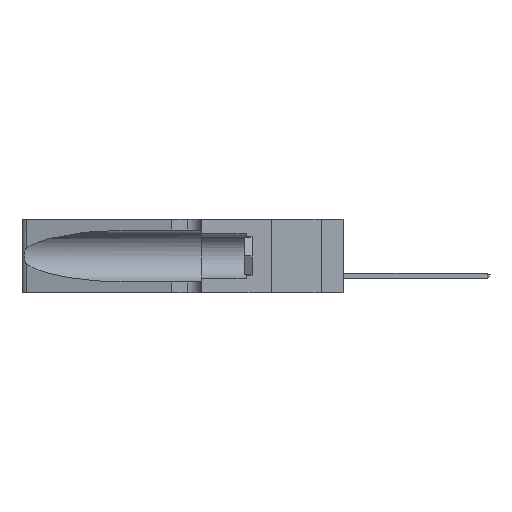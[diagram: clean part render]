
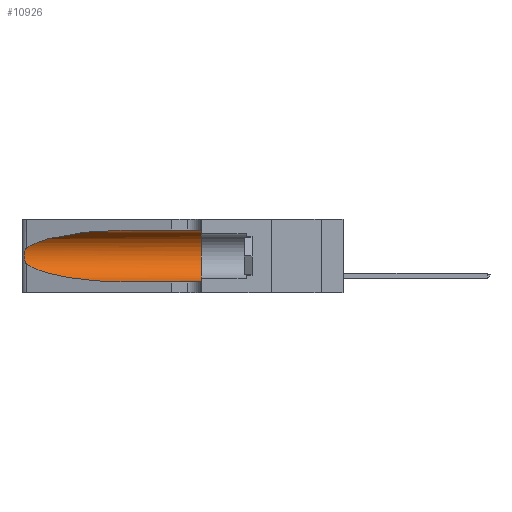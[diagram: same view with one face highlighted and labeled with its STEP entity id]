
A CAD part, left-side view. The second image highlights one B-rep face of the part: STEP entity #10926.
In plain terms, the highlighted cylindrical face has radius 3.308 mm (diameter 6.617 mm), a partial arc.
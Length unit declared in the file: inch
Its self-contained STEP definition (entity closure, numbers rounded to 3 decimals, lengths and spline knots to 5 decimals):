
#314 = EDGE_CURVE ( 'NONE', #3541, #20622, #6092, .T. ) ;
#514 = EDGE_CURVE ( 'NONE', #20622, #22971, #40554, .T. ) ;
#2762 = CARTESIAN_POINT ( 'NONE',  ( 0.1305, 0.35, 0.185 ) ) ;
#3541 = VERTEX_POINT ( 'NONE', #40699 ) ;
#4025 = EDGE_CURVE ( 'NONE', #7661, #39618, #10793, .T. ) ;
#6092 = B_SPLINE_CURVE_WITH_KNOTS ( 'NONE', 3,
 ( #36665, #26395, #43293, #23139, #19908, #23837, #10514, #21017, #37216, #24835, #27905, #31429, #14700, #34963 ),
 .UNSPECIFIED., .F., .F.,
 ( 4, 2, 2, 2, 2, 2, 4 ),
 ( 0., 0.00027, 0.00053, 0.00107, 0.0016, 0.00187, 0.00214 ),
 .UNSPECIFIED. ) ;
#6125 = ORIENTED_EDGE ( 'NONE', *, *, #314, .T. ) ;
#6126 = VERTEX_POINT ( 'NONE', #25216 ) ;
#7661 = VERTEX_POINT ( 'NONE', #43264 ) ;
#8004 = CARTESIAN_POINT ( 'NONE',  ( 0.18966, 0.96281, 0.31525 ) ) ;
#10514 = CARTESIAN_POINT ( 'NONE',  ( 0.26075, 1.23896, 0.19203 ) ) ;
#10696 = FACE_OUTER_BOUND ( 'NONE', #18994, .T. ) ;
#10793 = LINE ( 'NONE', #30307, #28112 ) ;
#10926 = ADVANCED_FACE ( 'NONE', ( #10696 ), #25385, .F. ) ;
#12500 = ORIENTED_EDGE ( 'NONE', *, *, #34162, .T. ) ;
#12620 = VECTOR ( 'NONE', #21405, 39.37008 ) ;
#12849 = CARTESIAN_POINT ( 'NONE',  ( 0.1305, 0.72297, 0.05475 ) ) ;
#13136 = ORIENTED_EDGE ( 'NONE', *, *, #28836, .F. ) ;
#13642 = LINE ( 'NONE', #21559, #12620 ) ;
#14700 = CARTESIAN_POINT ( 'NONE',  ( 0.25555, 1.22993, 0.14849 ) ) ;
#14718 = CIRCLE ( 'NONE', #21326, 0.13025 ) ;
#15798 = DIRECTION ( 'NONE',  ( 0., -1., 0. ) ) ;
#18134 = CARTESIAN_POINT ( 'NONE',  ( 0.2373, 1.15595, 0.28018 ) ) ;
#18273 = CARTESIAN_POINT ( 'NONE',  ( 0.1305, 0.72297, 0.31525 ) ) ;
#18450 =( BOUNDED_CURVE ( )  B_SPLINE_CURVE ( 3, ( #18273, #8004, #18134, #21507 ),
 .UNSPECIFIED., .F., .F. ) 
 B_SPLINE_CURVE_WITH_KNOTS ( ( 4, 4 ),
 ( 1.5708, 2.84003 ),
 .UNSPECIFIED. ) 
 CURVE ( )  GEOMETRIC_REPRESENTATION_ITEM ( )  RATIONAL_B_SPLINE_CURVE ( ( 1., 0.87, 0.87, 1. ) ) 
 REPRESENTATION_ITEM ( '' )  );
#18994 = EDGE_LOOP ( 'NONE', ( #28108, #6125, #21442, #12500, #13136, #21754 ) ) ;
#19150 = CARTESIAN_POINT ( 'NONE',  ( 0.1305, 1.61858, 0.185 ) ) ;
#19908 = CARTESIAN_POINT ( 'NONE',  ( 0.25854, 1.2359, 0.20912 ) ) ;
#20622 = VERTEX_POINT ( 'NONE', #31374 ) ;
#21017 = CARTESIAN_POINT ( 'NONE',  ( 0.26075, 1.23896, 0.178 ) ) ;
#21326 = AXIS2_PLACEMENT_3D ( 'NONE', #2762, #23644, #23902 ) ;
#21405 = DIRECTION ( 'NONE',  ( 0., -1., 0. ) ) ;
#21442 = ORIENTED_EDGE ( 'NONE', *, *, #514, .T. ) ;
#21507 = CARTESIAN_POINT ( 'NONE',  ( 0.25487, 1.22718, 0.22369 ) ) ;
#21559 = CARTESIAN_POINT ( 'NONE',  ( 0.1305, 1.61858, 0.05475 ) ) ;
#21754 = ORIENTED_EDGE ( 'NONE', *, *, #4025, .F. ) ;
#22971 = VERTEX_POINT ( 'NONE', #33405 ) ;
#23098 = CARTESIAN_POINT ( 'NONE',  ( 0.1305, 0.35, 0.31525 ) ) ;
#23139 = CARTESIAN_POINT ( 'NONE',  ( 0.25787, 1.23484, 0.2124 ) ) ;
#23644 = DIRECTION ( 'NONE',  ( 0., 1., 0. ) ) ;
#23837 = CARTESIAN_POINT ( 'NONE',  ( 0.26018, 1.23835, 0.19895 ) ) ;
#23902 = DIRECTION ( 'NONE',  ( 0., 0., 1. ) ) ;
#24835 = CARTESIAN_POINT ( 'NONE',  ( 0.25856, 1.23593, 0.16098 ) ) ;
#25216 = CARTESIAN_POINT ( 'NONE',  ( 0.1305, 0.35, 0.05475 ) ) ;
#25385 = CYLINDRICAL_SURFACE ( 'NONE', #34604, 0.13025 ) ;
#26223 = CARTESIAN_POINT ( 'NONE',  ( 0.18966, 0.96281, 0.05475 ) ) ;
#26395 = CARTESIAN_POINT ( 'NONE',  ( 0.25555, 1.22994, 0.2215 ) ) ;
#27905 = CARTESIAN_POINT ( 'NONE',  ( 0.25789, 1.23486, 0.15765 ) ) ;
#28108 = ORIENTED_EDGE ( 'NONE', *, *, #28659, .T. ) ;
#28112 = VECTOR ( 'NONE', #33716, 39.37008 ) ;
#28659 = EDGE_CURVE ( 'NONE', #7661, #3541, #18450, .T. ) ;
#28836 = EDGE_CURVE ( 'NONE', #39618, #6126, #14718, .T. ) ;
#30307 = CARTESIAN_POINT ( 'NONE',  ( 0.1305, 1.61858, 0.31525 ) ) ;
#31374 = CARTESIAN_POINT ( 'NONE',  ( 0.25487, 1.22718, 0.14631 ) ) ;
#31429 = CARTESIAN_POINT ( 'NONE',  ( 0.25639, 1.23186, 0.15144 ) ) ;
#32364 = DIRECTION ( 'NONE',  ( 0., 0., -1. ) ) ;
#33405 = CARTESIAN_POINT ( 'NONE',  ( 0.1305, 0.72297, 0.05475 ) ) ;
#33716 = DIRECTION ( 'NONE',  ( 0., -1., 0. ) ) ;
#34162 = EDGE_CURVE ( 'NONE', #22971, #6126, #13642, .T. ) ;
#34604 = AXIS2_PLACEMENT_3D ( 'NONE', #19150, #15798, #32364 ) ;
#34963 = CARTESIAN_POINT ( 'NONE',  ( 0.25487, 1.22718, 0.14631 ) ) ;
#36665 = CARTESIAN_POINT ( 'NONE',  ( 0.25487, 1.22718, 0.22369 ) ) ;
#37216 = CARTESIAN_POINT ( 'NONE',  ( 0.26017, 1.23833, 0.17102 ) ) ;
#39611 = CARTESIAN_POINT ( 'NONE',  ( 0.2373, 1.15595, 0.08982 ) ) ;
#39618 = VERTEX_POINT ( 'NONE', #23098 ) ;
#40053 = CARTESIAN_POINT ( 'NONE',  ( 0.25487, 1.22718, 0.14631 ) ) ;
#40554 =( BOUNDED_CURVE ( )  B_SPLINE_CURVE ( 3, ( #40053, #39611, #26223, #12849 ),
 .UNSPECIFIED., .F., .F. ) 
 B_SPLINE_CURVE_WITH_KNOTS ( ( 4, 4 ),
 ( 3.44316, 4.71239 ),
 .UNSPECIFIED. ) 
 CURVE ( )  GEOMETRIC_REPRESENTATION_ITEM ( )  RATIONAL_B_SPLINE_CURVE ( ( 1., 0.87, 0.87, 1. ) ) 
 REPRESENTATION_ITEM ( '' )  );
#40699 = CARTESIAN_POINT ( 'NONE',  ( 0.25487, 1.22718, 0.22369 ) ) ;
#43264 = CARTESIAN_POINT ( 'NONE',  ( 0.1305, 0.72297, 0.31525 ) ) ;
#43293 = CARTESIAN_POINT ( 'NONE',  ( 0.25639, 1.23184, 0.21858 ) ) ;
